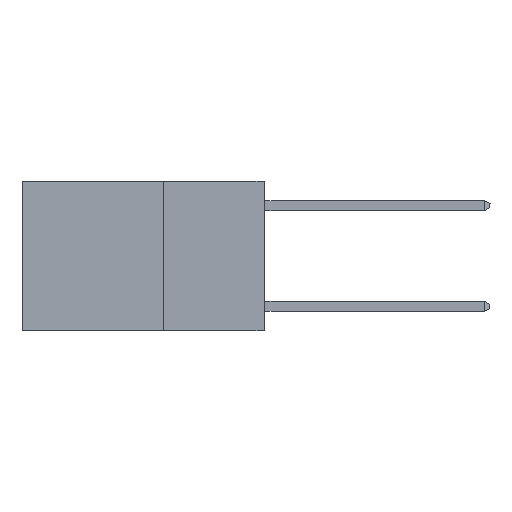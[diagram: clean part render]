
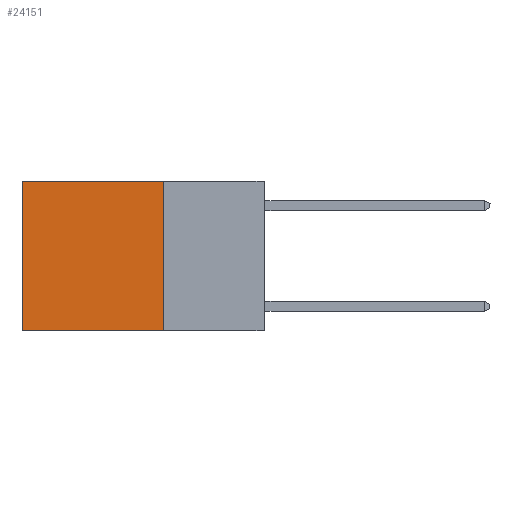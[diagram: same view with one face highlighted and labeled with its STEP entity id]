
A CAD part, left-side view. The second image highlights one B-rep face of the part: STEP entity #24151.
In plain terms, the highlighted planar face has unit normal (-1, 0, 0).
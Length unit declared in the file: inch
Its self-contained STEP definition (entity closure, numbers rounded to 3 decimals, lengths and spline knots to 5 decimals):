
#364 = ORIENTED_EDGE ( 'NONE', *, *, #8282, .F. ) ;
#1235 = CARTESIAN_POINT ( 'NONE',  ( 0.2625, 0.25, 0. ) ) ;
#3169 = VERTEX_POINT ( 'NONE', #30541 ) ;
#5015 = LINE ( 'NONE', #6907, #16170 ) ;
#5934 = ORIENTED_EDGE ( 'NONE', *, *, #22245, .T. ) ;
#6244 = DIRECTION ( 'NONE',  ( 0., 0., -1. ) ) ;
#6864 = EDGE_CURVE ( 'NONE', #3169, #10957, #6871, .T. ) ;
#6871 = LINE ( 'NONE', #13660, #27083 ) ;
#6907 = CARTESIAN_POINT ( 'NONE',  ( 0.2625, 0.6, 0. ) ) ;
#7550 = CARTESIAN_POINT ( 'NONE',  ( 0.2625, 0.6, -0.37 ) ) ;
#8282 = EDGE_CURVE ( 'NONE', #3169, #28960, #14096, .T. ) ;
#9734 = AXIS2_PLACEMENT_3D ( 'NONE', #31085, #21424, #18918 ) ;
#10460 = VERTEX_POINT ( 'NONE', #7550 ) ;
#10957 = VERTEX_POINT ( 'NONE', #31583 ) ;
#11419 = VECTOR ( 'NONE', #24993, 39.37008 ) ;
#13660 = CARTESIAN_POINT ( 'NONE',  ( 0.2625, 0.25, 0. ) ) ;
#14096 = LINE ( 'NONE', #1235, #27743 ) ;
#15443 = ORIENTED_EDGE ( 'NONE', *, *, #6864, .T. ) ;
#16170 = VECTOR ( 'NONE', #23983, 39.37008 ) ;
#16580 = PLANE ( 'NONE',  #9734 ) ;
#18918 = DIRECTION ( 'NONE',  ( 0., 0., -1. ) ) ;
#20735 = EDGE_LOOP ( 'NONE', ( #5934, #31263, #364, #15443 ) ) ;
#20954 = DIRECTION ( 'NONE',  ( 0., 1., 0. ) ) ;
#21424 = DIRECTION ( 'NONE',  ( 1., 0., 0. ) ) ;
#22245 = EDGE_CURVE ( 'NONE', #10957, #10460, #5015, .T. ) ;
#22417 = CARTESIAN_POINT ( 'NONE',  ( 0.2625, 0.25, -0.37 ) ) ;
#23793 = EDGE_CURVE ( 'NONE', #28960, #10460, #25164, .T. ) ;
#23983 = DIRECTION ( 'NONE',  ( 0., 0., -1. ) ) ;
#24151 = ADVANCED_FACE ( 'NONE', ( #27809 ), #16580, .F. ) ;
#24993 = DIRECTION ( 'NONE',  ( 0., 1., 0. ) ) ;
#25164 = LINE ( 'NONE', #22417, #11419 ) ;
#26499 = CARTESIAN_POINT ( 'NONE',  ( 0.2625, 0.25, -0.37 ) ) ;
#27083 = VECTOR ( 'NONE', #20954, 39.37008 ) ;
#27743 = VECTOR ( 'NONE', #6244, 39.37008 ) ;
#27809 = FACE_OUTER_BOUND ( 'NONE', #20735, .T. ) ;
#28960 = VERTEX_POINT ( 'NONE', #26499 ) ;
#30541 = CARTESIAN_POINT ( 'NONE',  ( 0.2625, 0.25, 0. ) ) ;
#31085 = CARTESIAN_POINT ( 'NONE',  ( 0.2625, 0.25, 0. ) ) ;
#31263 = ORIENTED_EDGE ( 'NONE', *, *, #23793, .F. ) ;
#31583 = CARTESIAN_POINT ( 'NONE',  ( 0.2625, 0.6, 0. ) ) ;
